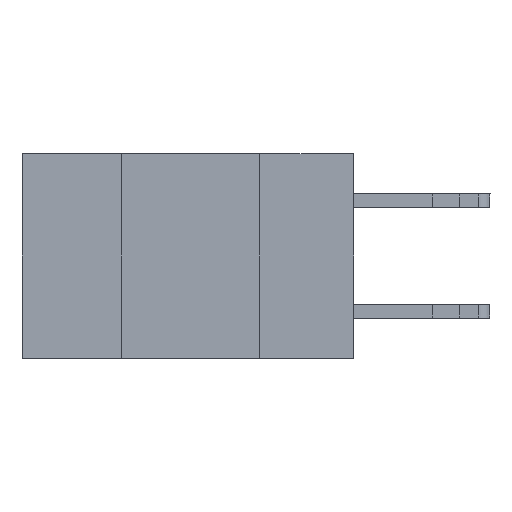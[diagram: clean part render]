
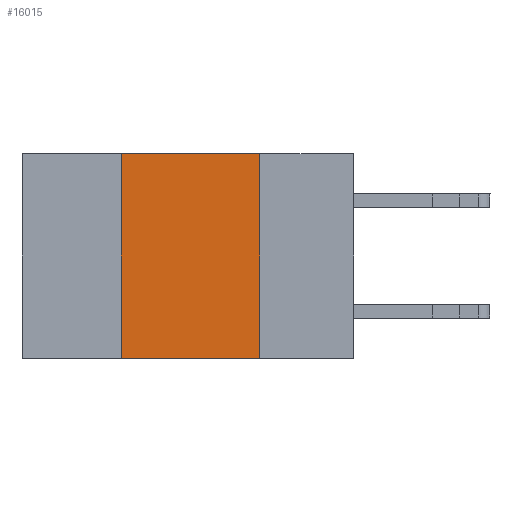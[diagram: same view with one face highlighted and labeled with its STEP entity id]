
A CAD part, left-side view. The second image highlights one B-rep face of the part: STEP entity #16015.
In plain terms, the highlighted planar face has unit normal (-1, 0, 0).
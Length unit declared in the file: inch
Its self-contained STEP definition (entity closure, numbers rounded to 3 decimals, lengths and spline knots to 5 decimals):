
#1123 = LINE ( 'NONE', #27843, #31885 ) ;
#1203 = VECTOR ( 'NONE', #21796, 39.37008 ) ;
#1338 = CARTESIAN_POINT ( 'NONE',  ( 0., 0.6, -0.37 ) ) ;
#3658 = ORIENTED_EDGE ( 'NONE', *, *, #21162, .F. ) ;
#3846 = LINE ( 'NONE', #1338, #1203 ) ;
#4407 = VERTEX_POINT ( 'NONE', #32828 ) ;
#6249 = VECTOR ( 'NONE', #23630, 39.37008 ) ;
#6586 = FACE_OUTER_BOUND ( 'NONE', #14943, .T. ) ;
#6812 = VERTEX_POINT ( 'NONE', #20725 ) ;
#8505 = LINE ( 'NONE', #27872, #6249 ) ;
#8825 = VECTOR ( 'NONE', #13555, 39.37008 ) ;
#9264 = LINE ( 'NONE', #19282, #8825 ) ;
#12192 = AXIS2_PLACEMENT_3D ( 'NONE', #13244, #13494, #35916 ) ;
#13244 = CARTESIAN_POINT ( 'NONE',  ( 0., 0.6, 0. ) ) ;
#13494 = DIRECTION ( 'NONE',  ( 1., 0., 0. ) ) ;
#13555 = DIRECTION ( 'NONE',  ( 0., -1., 0. ) ) ;
#14370 = EDGE_CURVE ( 'NONE', #4407, #15675, #3846, .T. ) ;
#14943 = EDGE_LOOP ( 'NONE', ( #28755, #16249, #3658, #20086 ) ) ;
#15536 = VERTEX_POINT ( 'NONE', #32519 ) ;
#15675 = VERTEX_POINT ( 'NONE', #17242 ) ;
#16015 = ADVANCED_FACE ( 'NONE', ( #6586 ), #19205, .F. ) ;
#16148 = DIRECTION ( 'NONE',  ( 0., 0., -1. ) ) ;
#16249 = ORIENTED_EDGE ( 'NONE', *, *, #22749, .F. ) ;
#17242 = CARTESIAN_POINT ( 'NONE',  ( 0., 0.17, -0.37 ) ) ;
#17405 = EDGE_CURVE ( 'NONE', #6812, #15675, #1123, .T. ) ;
#19205 = PLANE ( 'NONE',  #12192 ) ;
#19282 = CARTESIAN_POINT ( 'NONE',  ( 0., 0.6, 0. ) ) ;
#20086 = ORIENTED_EDGE ( 'NONE', *, *, #14370, .T. ) ;
#20725 = CARTESIAN_POINT ( 'NONE',  ( 0., 0.17, 0. ) ) ;
#21162 = EDGE_CURVE ( 'NONE', #4407, #15536, #8505, .T. ) ;
#21796 = DIRECTION ( 'NONE',  ( 0., -1., 0. ) ) ;
#22749 = EDGE_CURVE ( 'NONE', #15536, #6812, #9264, .T. ) ;
#23630 = DIRECTION ( 'NONE',  ( 0., 0., 1. ) ) ;
#27843 = CARTESIAN_POINT ( 'NONE',  ( 0., 0.17, 0. ) ) ;
#27872 = CARTESIAN_POINT ( 'NONE',  ( 0., 0.42, 0. ) ) ;
#28755 = ORIENTED_EDGE ( 'NONE', *, *, #17405, .F. ) ;
#31885 = VECTOR ( 'NONE', #16148, 39.37008 ) ;
#32519 = CARTESIAN_POINT ( 'NONE',  ( 0., 0.42, 0. ) ) ;
#32828 = CARTESIAN_POINT ( 'NONE',  ( 0., 0.42, -0.37 ) ) ;
#35916 = DIRECTION ( 'NONE',  ( 0., 0., -1. ) ) ;
